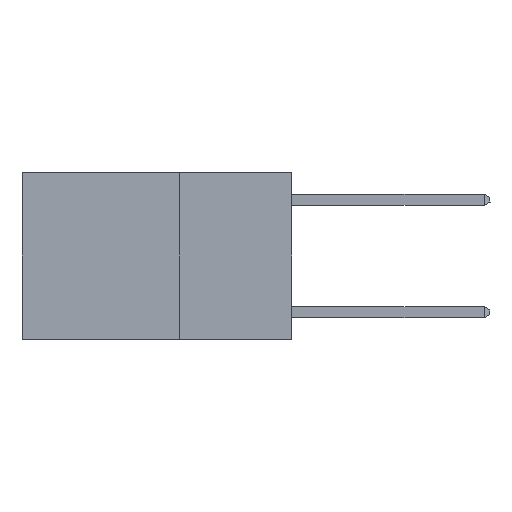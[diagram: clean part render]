
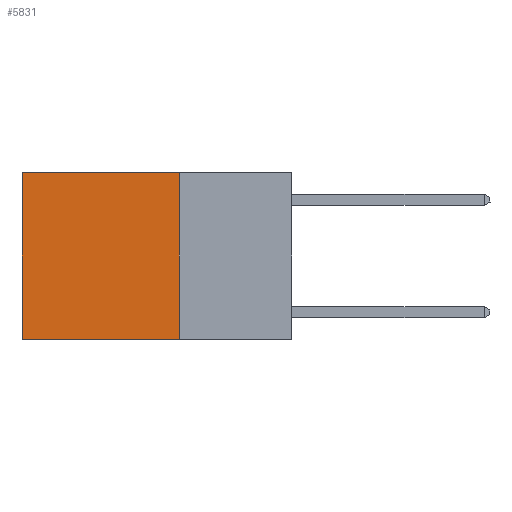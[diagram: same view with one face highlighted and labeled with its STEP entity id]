
A CAD part, left-side view. The second image highlights one B-rep face of the part: STEP entity #5831.
In plain terms, the highlighted planar face has unit normal (-1, 0, 0).
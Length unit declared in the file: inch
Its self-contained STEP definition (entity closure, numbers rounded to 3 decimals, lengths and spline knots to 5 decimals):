
#4 = DIRECTION ( 'NONE',  ( 0., 0., -1. ) ) ;
#550 = DIRECTION ( 'NONE',  ( 0., 1., 0. ) ) ;
#1298 = VECTOR ( 'NONE', #16304, 39.37008 ) ;
#1785 = VERTEX_POINT ( 'NONE', #8023 ) ;
#2141 = DIRECTION ( 'NONE',  ( 0., 0., -1. ) ) ;
#5545 = LINE ( 'NONE', #18771, #17965 ) ;
#5640 = EDGE_CURVE ( 'NONE', #18540, #14280, #20666, .T. ) ;
#5659 = CARTESIAN_POINT ( 'NONE',  ( 0.2625, 0.25, 0. ) ) ;
#5831 = ADVANCED_FACE ( 'NONE', ( #20329 ), #24237, .F. ) ;
#6185 = CARTESIAN_POINT ( 'NONE',  ( 0.2625, 0.6, 0. ) ) ;
#6841 = VERTEX_POINT ( 'NONE', #14685 ) ;
#7364 = AXIS2_PLACEMENT_3D ( 'NONE', #10130, #20514, #4 ) ;
#7802 = EDGE_CURVE ( 'NONE', #1785, #18540, #5545, .T. ) ;
#8023 = CARTESIAN_POINT ( 'NONE',  ( 0.2625, 0.25, 0. ) ) ;
#10130 = CARTESIAN_POINT ( 'NONE',  ( 0.2625, 0.25, 0. ) ) ;
#10277 = EDGE_LOOP ( 'NONE', ( #16154, #25557, #13117, #11274 ) ) ;
#10281 = CARTESIAN_POINT ( 'NONE',  ( 0.2625, 0.6, 0. ) ) ;
#11274 = ORIENTED_EDGE ( 'NONE', *, *, #7802, .T. ) ;
#12629 = DIRECTION ( 'NONE',  ( 0., 1., 0. ) ) ;
#13117 = ORIENTED_EDGE ( 'NONE', *, *, #14622, .F. ) ;
#14280 = VERTEX_POINT ( 'NONE', #15362 ) ;
#14622 = EDGE_CURVE ( 'NONE', #1785, #6841, #18536, .T. ) ;
#14685 = CARTESIAN_POINT ( 'NONE',  ( 0.2625, 0.25, -0.37 ) ) ;
#15197 = VECTOR ( 'NONE', #2141, 39.37008 ) ;
#15319 = VECTOR ( 'NONE', #12629, 39.37008 ) ;
#15362 = CARTESIAN_POINT ( 'NONE',  ( 0.2625, 0.6, -0.37 ) ) ;
#16154 = ORIENTED_EDGE ( 'NONE', *, *, #5640, .T. ) ;
#16304 = DIRECTION ( 'NONE',  ( 0., 0., -1. ) ) ;
#16895 = LINE ( 'NONE', #18157, #15319 ) ;
#17965 = VECTOR ( 'NONE', #550, 39.37008 ) ;
#18157 = CARTESIAN_POINT ( 'NONE',  ( 0.2625, 0.25, -0.37 ) ) ;
#18536 = LINE ( 'NONE', #5659, #1298 ) ;
#18540 = VERTEX_POINT ( 'NONE', #6185 ) ;
#18771 = CARTESIAN_POINT ( 'NONE',  ( 0.2625, 0.25, 0. ) ) ;
#20329 = FACE_OUTER_BOUND ( 'NONE', #10277, .T. ) ;
#20514 = DIRECTION ( 'NONE',  ( 1., 0., 0. ) ) ;
#20666 = LINE ( 'NONE', #10281, #15197 ) ;
#24237 = PLANE ( 'NONE',  #7364 ) ;
#24631 = EDGE_CURVE ( 'NONE', #6841, #14280, #16895, .T. ) ;
#25557 = ORIENTED_EDGE ( 'NONE', *, *, #24631, .F. ) ;
